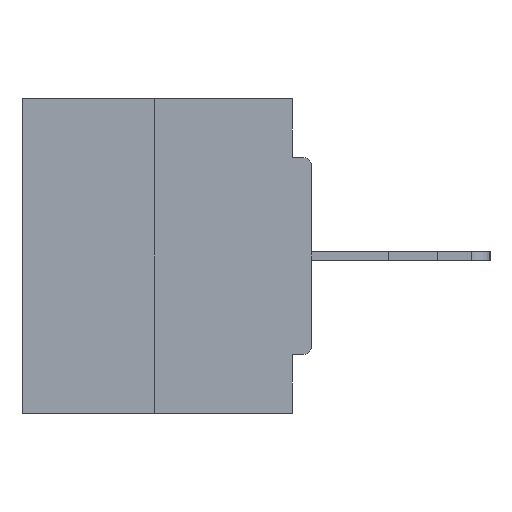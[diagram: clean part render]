
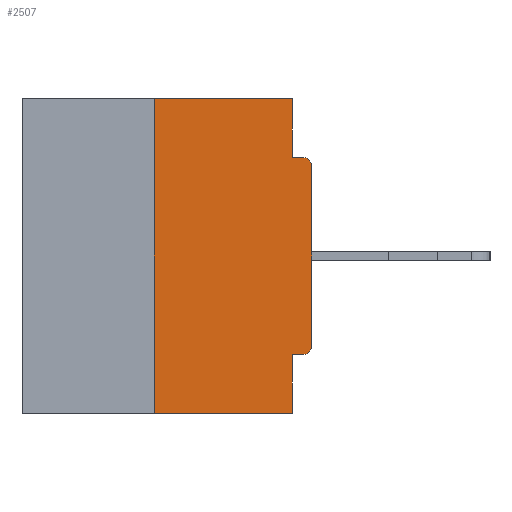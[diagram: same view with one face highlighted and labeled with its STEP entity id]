
A CAD part, left-side view. The second image highlights one B-rep face of the part: STEP entity #2507.
In plain terms, the highlighted planar face has unit normal (-1, 0, 0).
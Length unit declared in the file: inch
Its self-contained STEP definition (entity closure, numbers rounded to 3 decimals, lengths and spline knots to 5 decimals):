
#140 = AXIS2_PLACEMENT_3D ( 'NONE', #10653, #13055, #10486 ) ;
#182 = EDGE_CURVE ( 'NONE', #26850, #26415, #13987, .T. ) ;
#896 = LINE ( 'NONE', #10836, #23750 ) ;
#1080 = CARTESIAN_POINT ( 'NONE',  ( 0., 0.46, 0. ) ) ;
#1285 = CARTESIAN_POINT ( 'NONE',  ( 0., 0.031, 0. ) ) ;
#1365 = VERTEX_POINT ( 'NONE', #5346 ) ;
#1380 = VECTOR ( 'NONE', #25157, 39.37008 ) ;
#1542 = VERTEX_POINT ( 'NONE', #3576 ) ;
#1849 = EDGE_LOOP ( 'NONE', ( #16145, #20488, #26568, #25279, #30129, #9172, #12047, #14686, #25094, #8381 ) ) ;
#2507 = ADVANCED_FACE ( 'NONE', ( #7952 ), #20291, .F. ) ;
#2984 = CARTESIAN_POINT ( 'NONE',  ( 0., 0.015, -0.0935 ) ) ;
#3031 = LINE ( 'NONE', #10574, #1380 ) ;
#3044 = VECTOR ( 'NONE', #11070, 39.37008 ) ;
#3576 = CARTESIAN_POINT ( 'NONE',  ( 0., 0.25, -0.5 ) ) ;
#4060 = VECTOR ( 'NONE', #30364, 39.37008 ) ;
#4697 = CARTESIAN_POINT ( 'NONE',  ( 0., 0.015, -0.4065 ) ) ;
#4726 = CARTESIAN_POINT ( 'NONE',  ( 0., 0.25, 0. ) ) ;
#5346 = CARTESIAN_POINT ( 'NONE',  ( 0., 0.031, -0.4065 ) ) ;
#7743 = CARTESIAN_POINT ( 'NONE',  ( 0., 0., -0.1085 ) ) ;
#7801 = VERTEX_POINT ( 'NONE', #17921 ) ;
#7952 = FACE_OUTER_BOUND ( 'NONE', #1849, .T. ) ;
#8110 = LINE ( 'NONE', #25424, #13416 ) ;
#8115 = DIRECTION ( 'NONE',  ( 1., 0., 0. ) ) ;
#8381 = ORIENTED_EDGE ( 'NONE', *, *, #13340, .F. ) ;
#9172 = ORIENTED_EDGE ( 'NONE', *, *, #28269, .T. ) ;
#9634 = CARTESIAN_POINT ( 'NONE',  ( 0., 0., -0.0935 ) ) ;
#10221 = CARTESIAN_POINT ( 'NONE',  ( 0., 0., -0.3915 ) ) ;
#10427 = VERTEX_POINT ( 'NONE', #10221 ) ;
#10486 = DIRECTION ( 'NONE',  ( 0., 0., -1. ) ) ;
#10574 = CARTESIAN_POINT ( 'NONE',  ( 0., 0.46, -0.5 ) ) ;
#10653 = CARTESIAN_POINT ( 'NONE',  ( 0., 0.015, -0.1085 ) ) ;
#10836 = CARTESIAN_POINT ( 'NONE',  ( 0., 0.031, -0.5 ) ) ;
#11070 = DIRECTION ( 'NONE',  ( 0., 0., -1. ) ) ;
#11733 = EDGE_CURVE ( 'NONE', #7801, #26415, #12349, .T. ) ;
#12047 = ORIENTED_EDGE ( 'NONE', *, *, #17276, .T. ) ;
#12349 = LINE ( 'NONE', #9634, #25006 ) ;
#12520 = VERTEX_POINT ( 'NONE', #4697 ) ;
#13055 = DIRECTION ( 'NONE',  ( -1., 0., 0. ) ) ;
#13340 = EDGE_CURVE ( 'NONE', #22239, #7801, #13464, .T. ) ;
#13416 = VECTOR ( 'NONE', #30259, 39.37008 ) ;
#13464 = LINE ( 'NONE', #1285, #3044 ) ;
#13987 = CIRCLE ( 'NONE', #140, 0.015 ) ;
#14686 = ORIENTED_EDGE ( 'NONE', *, *, #182, .T. ) ;
#15893 = LINE ( 'NONE', #25685, #4060 ) ;
#15940 = DIRECTION ( 'NONE',  ( 0., 0., -1. ) ) ;
#16104 = CARTESIAN_POINT ( 'NONE',  ( 0., 0.031, -0.5 ) ) ;
#16145 = ORIENTED_EDGE ( 'NONE', *, *, #20428, .F. ) ;
#16243 = DIRECTION ( 'NONE',  ( 0., 0., -1. ) ) ;
#16726 = EDGE_CURVE ( 'NONE', #1542, #29641, #8110, .T. ) ;
#17276 = EDGE_CURVE ( 'NONE', #10427, #26850, #27959, .T. ) ;
#17921 = CARTESIAN_POINT ( 'NONE',  ( 0., 0.031, -0.0935 ) ) ;
#18810 = CARTESIAN_POINT ( 'NONE',  ( 0., 0.015, -0.3915 ) ) ;
#19643 = EDGE_CURVE ( 'NONE', #12520, #1365, #15893, .T. ) ;
#20291 = PLANE ( 'NONE',  #25716 ) ;
#20428 = EDGE_CURVE ( 'NONE', #29641, #22239, #23040, .T. ) ;
#20488 = ORIENTED_EDGE ( 'NONE', *, *, #16726, .F. ) ;
#20567 = CARTESIAN_POINT ( 'NONE',  ( 0., 0., 0. ) ) ;
#22239 = VERTEX_POINT ( 'NONE', #27730 ) ;
#23040 = LINE ( 'NONE', #1080, #24090 ) ;
#23750 = VECTOR ( 'NONE', #15940, 39.37008 ) ;
#24090 = VECTOR ( 'NONE', #28024, 39.37008 ) ;
#24478 = VERTEX_POINT ( 'NONE', #16104 ) ;
#24958 = DIRECTION ( 'NONE',  ( 0., 0., -1. ) ) ;
#25006 = VECTOR ( 'NONE', #31305, 39.37008 ) ;
#25094 = ORIENTED_EDGE ( 'NONE', *, *, #11733, .F. ) ;
#25157 = DIRECTION ( 'NONE',  ( 0., -1., 0. ) ) ;
#25279 = ORIENTED_EDGE ( 'NONE', *, *, #25636, .F. ) ;
#25424 = CARTESIAN_POINT ( 'NONE',  ( 0., 0.25, 0. ) ) ;
#25636 = EDGE_CURVE ( 'NONE', #1365, #24478, #896, .T. ) ;
#25685 = CARTESIAN_POINT ( 'NONE',  ( 0., 0., -0.4065 ) ) ;
#25716 = AXIS2_PLACEMENT_3D ( 'NONE', #30100, #8115, #24958 ) ;
#26415 = VERTEX_POINT ( 'NONE', #2984 ) ;
#26568 = ORIENTED_EDGE ( 'NONE', *, *, #28929, .T. ) ;
#26850 = VERTEX_POINT ( 'NONE', #7743 ) ;
#27258 = VECTOR ( 'NONE', #28431, 39.37008 ) ;
#27461 = AXIS2_PLACEMENT_3D ( 'NONE', #18810, #28127, #16243 ) ;
#27730 = CARTESIAN_POINT ( 'NONE',  ( 0., 0.031, 0. ) ) ;
#27959 = LINE ( 'NONE', #20567, #27258 ) ;
#28024 = DIRECTION ( 'NONE',  ( 0., -1., 0. ) ) ;
#28127 = DIRECTION ( 'NONE',  ( -1., 0., 0. ) ) ;
#28269 = EDGE_CURVE ( 'NONE', #12520, #10427, #31578, .T. ) ;
#28431 = DIRECTION ( 'NONE',  ( 0., 0., 1. ) ) ;
#28929 = EDGE_CURVE ( 'NONE', #1542, #24478, #3031, .T. ) ;
#29641 = VERTEX_POINT ( 'NONE', #4726 ) ;
#30100 = CARTESIAN_POINT ( 'NONE',  ( 0., 0.46, 0. ) ) ;
#30129 = ORIENTED_EDGE ( 'NONE', *, *, #19643, .F. ) ;
#30259 = DIRECTION ( 'NONE',  ( 0., 0., 1. ) ) ;
#30364 = DIRECTION ( 'NONE',  ( 0., 1., 0. ) ) ;
#31305 = DIRECTION ( 'NONE',  ( 0., -1., 0. ) ) ;
#31578 = CIRCLE ( 'NONE', #27461, 0.015 ) ;
